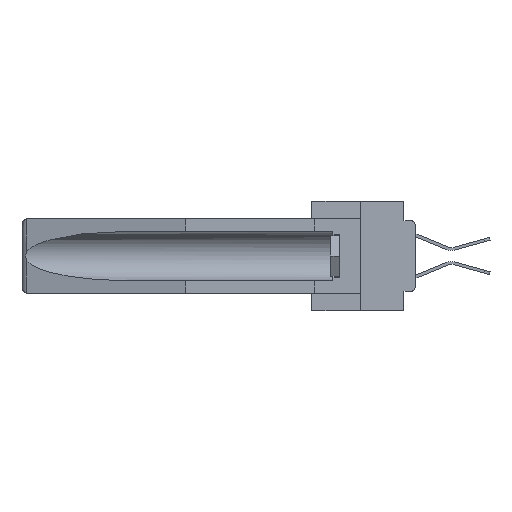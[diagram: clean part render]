
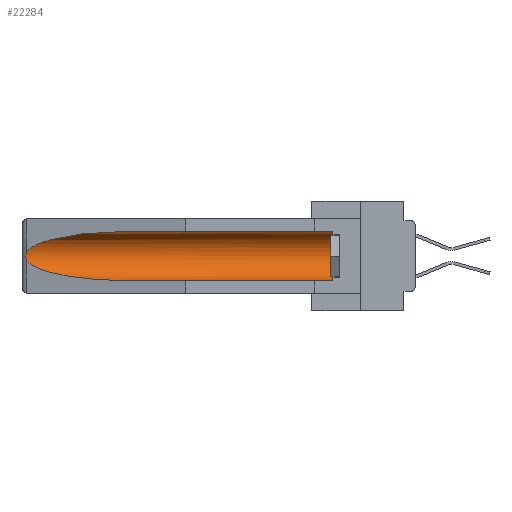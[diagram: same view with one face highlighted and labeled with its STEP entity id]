
A CAD part, left-side view. The second image highlights one B-rep face of the part: STEP entity #22284.
In plain terms, the highlighted cylindrical face has radius 2.857 mm (diameter 5.715 mm), a partial arc.
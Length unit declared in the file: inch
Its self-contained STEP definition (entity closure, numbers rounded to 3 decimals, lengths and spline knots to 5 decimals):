
#346 = LINE ( 'NONE', #14225, #33217 ) ;
#910 = DIRECTION ( 'NONE',  ( 0., 1., 0. ) ) ;
#1169 = CARTESIAN_POINT ( 'NONE',  ( 0.2673, 1.53269, -0.17917 ) ) ;
#1472 = CARTESIAN_POINT ( 'NONE',  ( 0.155, 1.07973, -0.059 ) ) ;
#1939 = VERTEX_POINT ( 'NONE', #4501 ) ;
#2608 = VERTEX_POINT ( 'NONE', #1472 ) ;
#3146 = EDGE_CURVE ( 'NONE', #27982, #31990, #6453, .T. ) ;
#3703 = EDGE_CURVE ( 'NONE', #2608, #16913, #6229, .T. ) ;
#4126 = EDGE_CURVE ( 'NONE', #16913, #27982, #7438, .T. ) ;
#4165 = CARTESIAN_POINT ( 'NONE',  ( 0.26537, 1.52718, -0.19328 ) ) ;
#4501 = CARTESIAN_POINT ( 'NONE',  ( 0.155, 0.126, -0.284 ) ) ;
#4601 = CARTESIAN_POINT ( 'NONE',  ( 0.26655, 1.53094, -0.18657 ) ) ;
#5277 = DIRECTION ( 'NONE',  ( 0., -1., 0. ) ) ;
#5892 = EDGE_CURVE ( 'NONE', #1939, #31990, #31729, .T. ) ;
#6229 =( BOUNDED_CURVE ( )  B_SPLINE_CURVE ( 3, ( #15266, #13065, #15809, #27173 ),
 .UNSPECIFIED., .F., .F. ) 
 B_SPLINE_CURVE_WITH_KNOTS ( ( 4, 4 ),
 ( 4.71239, 6.08839 ),
 .UNSPECIFIED. ) 
 CURVE ( )  GEOMETRIC_REPRESENTATION_ITEM ( )  RATIONAL_B_SPLINE_CURVE ( ( 1., 0.848, 0.848, 1. ) ) 
 REPRESENTATION_ITEM ( '' )  );
#6453 =( BOUNDED_CURVE ( )  B_SPLINE_CURVE ( 3, ( #4165, #9645, #20824, #12045 ),
 .UNSPECIFIED., .F., .F. ) 
 B_SPLINE_CURVE_WITH_KNOTS ( ( 4, 4 ),
 ( 0.1948, 1.5708 ),
 .UNSPECIFIED. ) 
 CURVE ( )  GEOMETRIC_REPRESENTATION_ITEM ( )  RATIONAL_B_SPLINE_CURVE ( ( 1., 0.848, 0.848, 1. ) ) 
 REPRESENTATION_ITEM ( '' )  );
#7179 = CARTESIAN_POINT ( 'NONE',  ( 0.26537, 1.52718, -0.14972 ) ) ;
#7438 = B_SPLINE_CURVE_WITH_KNOTS ( 'NONE', 3,
 ( #7179, #20738, #32603, #17975, #9564, #12655, #1169, #4601, #23847, #26414 ),
 .UNSPECIFIED., .F., .F.,
 ( 4, 2, 2, 2, 4 ),
 ( 0., 0.00029, 0.00058, 0.00087, 0.00117 ),
 .UNSPECIFIED. ) ;
#7895 = CARTESIAN_POINT ( 'NONE',  ( 0.26537, 1.52718, -0.14972 ) ) ;
#8878 = VERTEX_POINT ( 'NONE', #28286 ) ;
#8925 = DIRECTION ( 'NONE',  ( 0., 1., 0. ) ) ;
#9131 = VECTOR ( 'NONE', #32072, 39.37008 ) ;
#9545 = CARTESIAN_POINT ( 'NONE',  ( 0.155, 1.07973, -0.284 ) ) ;
#9564 = CARTESIAN_POINT ( 'NONE',  ( 0.2675, 1.53308, -0.16763 ) ) ;
#9645 = CARTESIAN_POINT ( 'NONE',  ( 0.25451, 1.48313, -0.24835 ) ) ;
#10578 = CARTESIAN_POINT ( 'NONE',  ( 0.155, 0.126, -0.1715 ) ) ;
#11323 = CARTESIAN_POINT ( 'NONE',  ( 0.155, -0.30754, -0.1715 ) ) ;
#11421 = CARTESIAN_POINT ( 'NONE',  ( 0.26537, 1.52718, -0.19328 ) ) ;
#12036 = AXIS2_PLACEMENT_3D ( 'NONE', #11323, #910, #14799 ) ;
#12045 = CARTESIAN_POINT ( 'NONE',  ( 0.155, 1.07973, -0.284 ) ) ;
#12448 = AXIS2_PLACEMENT_3D ( 'NONE', #10578, #5277, #29983 ) ;
#12655 = CARTESIAN_POINT ( 'NONE',  ( 0.2675, 1.53308, -0.17534 ) ) ;
#13065 = CARTESIAN_POINT ( 'NONE',  ( 0.21114, 1.30732, -0.059 ) ) ;
#13886 = ORIENTED_EDGE ( 'NONE', *, *, #5892, .F. ) ;
#14225 = CARTESIAN_POINT ( 'NONE',  ( 0.155, -0.30754, -0.059 ) ) ;
#14799 = DIRECTION ( 'NONE',  ( 0., 0., 1. ) ) ;
#15266 = CARTESIAN_POINT ( 'NONE',  ( 0.155, 1.07973, -0.059 ) ) ;
#15474 = EDGE_CURVE ( 'NONE', #1939, #8878, #23021, .T. ) ;
#15809 = CARTESIAN_POINT ( 'NONE',  ( 0.25451, 1.48313, -0.09465 ) ) ;
#16913 = VERTEX_POINT ( 'NONE', #7895 ) ;
#17975 = CARTESIAN_POINT ( 'NONE',  ( 0.2673, 1.5327, -0.16383 ) ) ;
#20738 = CARTESIAN_POINT ( 'NONE',  ( 0.26597, 1.52961, -0.15275 ) ) ;
#20824 = CARTESIAN_POINT ( 'NONE',  ( 0.21114, 1.30732, -0.284 ) ) ;
#22284 = ADVANCED_FACE ( 'NONE', ( #28181 ), #27994, .F. ) ;
#23021 = CIRCLE ( 'NONE', #12448, 0.1125 ) ;
#23060 = EDGE_LOOP ( 'NONE', ( #26970, #33149, #23874, #13886, #25454, #33488 ) ) ;
#23847 = CARTESIAN_POINT ( 'NONE',  ( 0.26597, 1.5296, -0.19026 ) ) ;
#23874 = ORIENTED_EDGE ( 'NONE', *, *, #3146, .T. ) ;
#25454 = ORIENTED_EDGE ( 'NONE', *, *, #15474, .T. ) ;
#26414 = CARTESIAN_POINT ( 'NONE',  ( 0.26537, 1.52718, -0.19328 ) ) ;
#26970 = ORIENTED_EDGE ( 'NONE', *, *, #3703, .T. ) ;
#27173 = CARTESIAN_POINT ( 'NONE',  ( 0.26537, 1.52718, -0.14972 ) ) ;
#27982 = VERTEX_POINT ( 'NONE', #11421 ) ;
#27994 = CYLINDRICAL_SURFACE ( 'NONE', #12036, 0.1125 ) ;
#28181 = FACE_OUTER_BOUND ( 'NONE', #23060, .T. ) ;
#28286 = CARTESIAN_POINT ( 'NONE',  ( 0.155, 0.126, -0.059 ) ) ;
#29983 = DIRECTION ( 'NONE',  ( 0., 0., 1. ) ) ;
#31729 = LINE ( 'NONE', #34284, #9131 ) ;
#31990 = VERTEX_POINT ( 'NONE', #9545 ) ;
#32072 = DIRECTION ( 'NONE',  ( 0., 1., 0. ) ) ;
#32603 = CARTESIAN_POINT ( 'NONE',  ( 0.26654, 1.53092, -0.15636 ) ) ;
#32639 = EDGE_CURVE ( 'NONE', #8878, #2608, #346, .T. ) ;
#33149 = ORIENTED_EDGE ( 'NONE', *, *, #4126, .T. ) ;
#33217 = VECTOR ( 'NONE', #8925, 39.37008 ) ;
#33488 = ORIENTED_EDGE ( 'NONE', *, *, #32639, .T. ) ;
#34284 = CARTESIAN_POINT ( 'NONE',  ( 0.155, -0.30754, -0.284 ) ) ;
